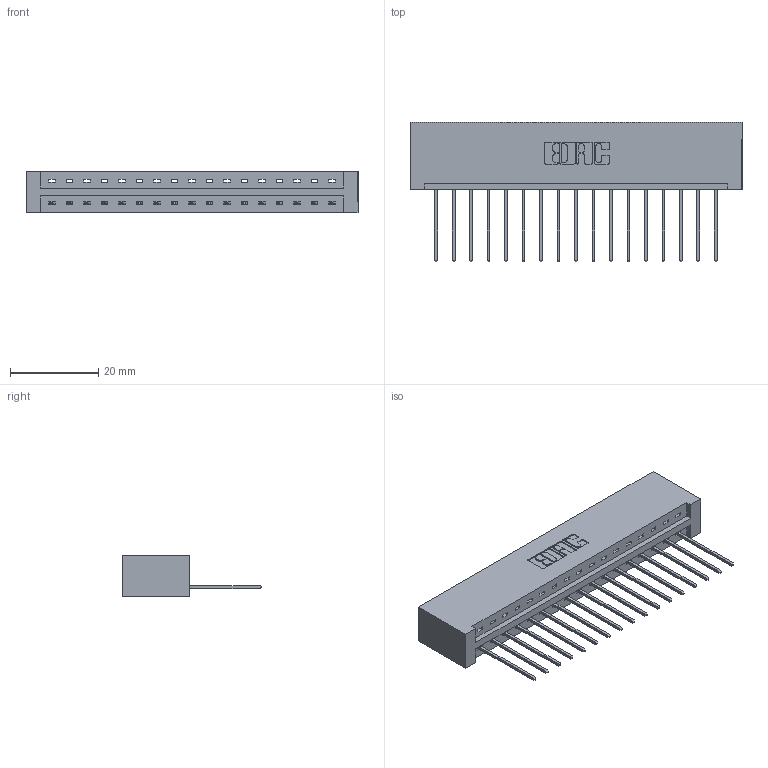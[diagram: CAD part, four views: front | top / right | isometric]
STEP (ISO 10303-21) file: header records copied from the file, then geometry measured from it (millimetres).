
FILE_DESCRIPTION (( 'STEP AP203' ), '1' );
FILE_NAME ('337-017-542-101.STEP', '2018-08-04T22:14:00', ( '' ), ( '' ), 'SwSTEP 2.0', 'SolidWorks 2016', '' );
FILE_SCHEMA (( 'CONFIG_CONTROL_DESIGN' ));
Length unit declared in the file: inch
Products named in the file (3): 337 Part_No Mounting Lugs; 345-292-001_345-293-142; 337-017-542-101
Assembly tree (18 placements, depth 2):
  337-017-542-101
    337 Part_No Mounting Lugs
    345-292-001_345-293-142  x17
Bounding box: 75.23 x 31.63 x 9.4 mm (x, y, z)
Volume: 8283.1 mm3; surface area: 8650.8 mm2
Topology: 18 solids, 18 shells, 1160 faces, 3483 edges, 2298 vertices
Faces by surface type: plane 848, cylinder 312
Entity records: 15611 total; most frequent: CARTESIAN_POINT 2725, ORIENTED_EDGE 2678, DIRECTION 2337, EDGE_CURVE 1339, VECTOR 1219, LINE 1219, VERTEX_POINT 890, AXIS2_PLACEMENT_3D 559
